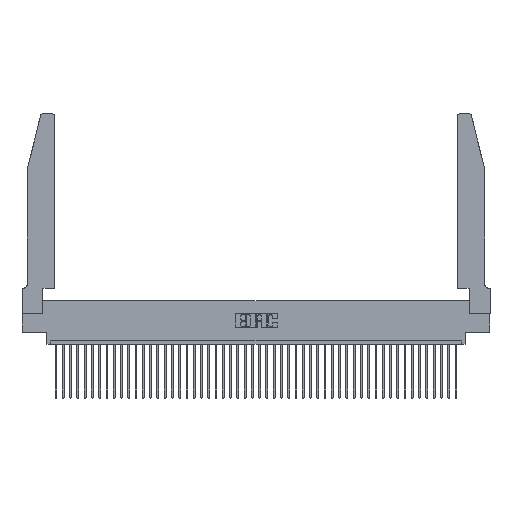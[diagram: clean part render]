
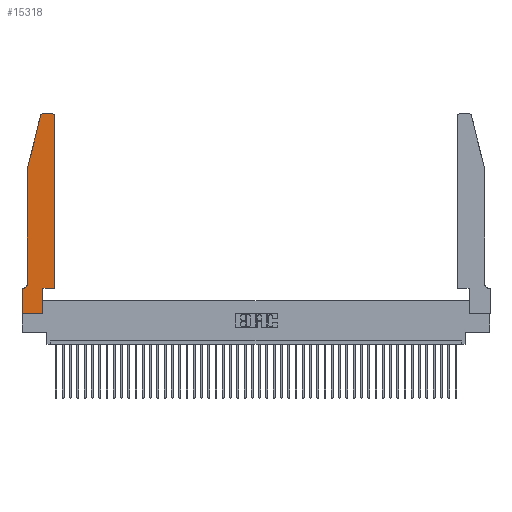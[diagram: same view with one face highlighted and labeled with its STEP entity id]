
A CAD part, top view. The second image highlights one B-rep face of the part: STEP entity #15318.
In plain terms, the highlighted planar face has unit normal (0, 0, 1).
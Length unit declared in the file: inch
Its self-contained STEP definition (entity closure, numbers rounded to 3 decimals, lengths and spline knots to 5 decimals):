
#3 = DIRECTION ( 'NONE',  ( 0., 1., 0. ) ) ;
#932 = DIRECTION ( 'NONE',  ( 0., -1., 0. ) ) ;
#965 = VECTOR ( 'NONE', #3, 39.37008 ) ;
#1330 = VERTEX_POINT ( 'NONE', #4524 ) ;
#2047 = ORIENTED_EDGE ( 'NONE', *, *, #10478, .T. ) ;
#2260 = LINE ( 'NONE', #42080, #41543 ) ;
#3039 = ORIENTED_EDGE ( 'NONE', *, *, #27211, .T. ) ;
#3111 = VERTEX_POINT ( 'NONE', #19077 ) ;
#3651 = LINE ( 'NONE', #14438, #29190 ) ;
#3782 = ORIENTED_EDGE ( 'NONE', *, *, #40038, .T. ) ;
#4115 = CARTESIAN_POINT ( 'NONE',  ( 0.0055, 0.35, 0.37 ) ) ;
#4524 = CARTESIAN_POINT ( 'NONE',  ( 0.25487, 2.72718, 0.37 ) ) ;
#4944 = EDGE_CURVE ( 'NONE', #32134, #42219, #15332, .T. ) ;
#6079 = CARTESIAN_POINT ( 'NONE',  ( 0.0755, 2., 0.37 ) ) ;
#6484 = EDGE_CURVE ( 'NONE', #40848, #12326, #9404, .T. ) ;
#7532 = CARTESIAN_POINT ( 'NONE',  ( 0.4505, 0.35, 0.37 ) ) ;
#8076 = DIRECTION ( 'NONE',  ( 0., 0., 1. ) ) ;
#8803 = ORIENTED_EDGE ( 'NONE', *, *, #30537, .T. ) ;
#9305 = ORIENTED_EDGE ( 'NONE', *, *, #6484, .T. ) ;
#9404 = LINE ( 'NONE', #20370, #38803 ) ;
#9510 = VERTEX_POINT ( 'NONE', #31432 ) ;
#9605 = CARTESIAN_POINT ( 'NONE',  ( 0.0055, 0.42, 0.37 ) ) ;
#9647 = VERTEX_POINT ( 'NONE', #38100 ) ;
#9669 = VECTOR ( 'NONE', #932, 39.37008 ) ;
#10478 = EDGE_CURVE ( 'NONE', #34378, #34641, #13978, .T. ) ;
#11453 = AXIS2_PLACEMENT_3D ( 'NONE', #23658, #41322, #34464 ) ;
#12167 = ORIENTED_EDGE ( 'NONE', *, *, #37083, .T. ) ;
#12326 = VERTEX_POINT ( 'NONE', #33422 ) ;
#13372 = CARTESIAN_POINT ( 'NONE',  ( 0., 0., 0.37 ) ) ;
#13695 = VECTOR ( 'NONE', #34147, 39.37008 ) ;
#13743 = ORIENTED_EDGE ( 'NONE', *, *, #31569, .T. ) ;
#13949 = DIRECTION ( 'NONE',  ( 0., 1., 0. ) ) ;
#13978 = CIRCLE ( 'NONE', #39617, 0.03 ) ;
#13996 = DIRECTION ( 'NONE',  ( 1., 0., 0. ) ) ;
#14005 = CARTESIAN_POINT ( 'NONE',  ( 0.2605, 2.75, 0.37 ) ) ;
#14438 = CARTESIAN_POINT ( 'NONE',  ( 0.0755, 2., 0.37 ) ) ;
#15318 = ADVANCED_FACE ( 'NONE', ( #31512 ), #33857, .T. ) ;
#15332 = LINE ( 'NONE', #20928, #13695 ) ;
#15644 = AXIS2_PLACEMENT_3D ( 'NONE', #9605, #44278, #34069 ) ;
#16637 = DIRECTION ( 'NONE',  ( 1., 0., 0. ) ) ;
#18770 = DIRECTION ( 'NONE',  ( 0., 0., 1. ) ) ;
#19077 = CARTESIAN_POINT ( 'NONE',  ( 0.284, 2.75, 0.37 ) ) ;
#20370 = CARTESIAN_POINT ( 'NONE',  ( 0.0755, 0.35, 0.37 ) ) ;
#20928 = CARTESIAN_POINT ( 'NONE',  ( 0., 0., 0.37 ) ) ;
#20960 = DIRECTION ( 'NONE',  ( -0.239, -0.971, 0. ) ) ;
#21564 = CARTESIAN_POINT ( 'NONE',  ( 0.284, 2.72, 0.37 ) ) ;
#21651 = CARTESIAN_POINT ( 'NONE',  ( 0.2865, 0.35, 0.37 ) ) ;
#22171 = LINE ( 'NONE', #35813, #9669 ) ;
#22509 = CARTESIAN_POINT ( 'NONE',  ( 0.4505, 2.72, 0.37 ) ) ;
#23502 = EDGE_CURVE ( 'NONE', #9510, #34378, #36922, .T. ) ;
#23594 = VECTOR ( 'NONE', #24025, 39.37008 ) ;
#23658 = CARTESIAN_POINT ( 'NONE',  ( 0., 0.35, 0.37 ) ) ;
#23957 = ORIENTED_EDGE ( 'NONE', *, *, #23502, .T. ) ;
#24025 = DIRECTION ( 'NONE',  ( -1., 0., 0. ) ) ;
#24248 = EDGE_CURVE ( 'NONE', #3111, #1330, #43454, .T. ) ;
#24462 = EDGE_CURVE ( 'NONE', #12326, #32134, #43469, .T. ) ;
#27211 = EDGE_CURVE ( 'NONE', #34641, #3111, #34525, .T. ) ;
#28226 = ORIENTED_EDGE ( 'NONE', *, *, #24248, .T. ) ;
#28287 = AXIS2_PLACEMENT_3D ( 'NONE', #21564, #18770, #16637 ) ;
#28865 = ORIENTED_EDGE ( 'NONE', *, *, #38122, .T. ) ;
#29190 = VECTOR ( 'NONE', #20960, 39.37008 ) ;
#30383 = CIRCLE ( 'NONE', #15644, 0.07 ) ;
#30537 = EDGE_CURVE ( 'NONE', #1330, #41046, #3651, .T. ) ;
#31432 = CARTESIAN_POINT ( 'NONE',  ( 0.4505, 0.35, 0.37 ) ) ;
#31512 = FACE_OUTER_BOUND ( 'NONE', #39662, .T. ) ;
#31569 = EDGE_CURVE ( 'NONE', #9647, #40848, #30383, .T. ) ;
#31606 = CARTESIAN_POINT ( 'NONE',  ( 0., 0., 0.37 ) ) ;
#32134 = VERTEX_POINT ( 'NONE', #13372 ) ;
#32686 = CARTESIAN_POINT ( 'NONE',  ( 0.4205, 2.72, 0.37 ) ) ;
#33422 = CARTESIAN_POINT ( 'NONE',  ( 0., 0.35, 0.37 ) ) ;
#33857 = PLANE ( 'NONE',  #11453 ) ;
#34069 = DIRECTION ( 'NONE',  ( -1., 0., 0. ) ) ;
#34147 = DIRECTION ( 'NONE',  ( 1., 0., 0. ) ) ;
#34378 = VERTEX_POINT ( 'NONE', #22509 ) ;
#34464 = DIRECTION ( 'NONE',  ( 1., 0., 0. ) ) ;
#34525 = LINE ( 'NONE', #14005, #23594 ) ;
#34641 = VERTEX_POINT ( 'NONE', #41523 ) ;
#34787 = VECTOR ( 'NONE', #39344, 39.37008 ) ;
#35813 = CARTESIAN_POINT ( 'NONE',  ( 0.0755, 2., 0.37 ) ) ;
#35886 = VERTEX_POINT ( 'NONE', #21651 ) ;
#36704 = ORIENTED_EDGE ( 'NONE', *, *, #24462, .T. ) ;
#36922 = LINE ( 'NONE', #7532, #965 ) ;
#37083 = EDGE_CURVE ( 'NONE', #41046, #9647, #22171, .T. ) ;
#37805 = CARTESIAN_POINT ( 'NONE',  ( 0.2865, 0., 0.37 ) ) ;
#38100 = CARTESIAN_POINT ( 'NONE',  ( 0.0755, 0.42, 0.37 ) ) ;
#38122 = EDGE_CURVE ( 'NONE', #35886, #9510, #42827, .T. ) ;
#38803 = VECTOR ( 'NONE', #41361, 39.37008 ) ;
#39344 = DIRECTION ( 'NONE',  ( 0., -1., 0. ) ) ;
#39617 = AXIS2_PLACEMENT_3D ( 'NONE', #32686, #8076, #39830 ) ;
#39662 = EDGE_LOOP ( 'NONE', ( #3039, #28226, #8803, #12167, #13743, #9305, #36704, #40674, #3782, #28865, #23957, #2047 ) ) ;
#39830 = DIRECTION ( 'NONE',  ( 1., 0., 0. ) ) ;
#40038 = EDGE_CURVE ( 'NONE', #42219, #35886, #2260, .T. ) ;
#40638 = VECTOR ( 'NONE', #13996, 39.37008 ) ;
#40674 = ORIENTED_EDGE ( 'NONE', *, *, #4944, .T. ) ;
#40848 = VERTEX_POINT ( 'NONE', #4115 ) ;
#41046 = VERTEX_POINT ( 'NONE', #6079 ) ;
#41322 = DIRECTION ( 'NONE',  ( 0., 0., 1. ) ) ;
#41361 = DIRECTION ( 'NONE',  ( -1., 0., 0. ) ) ;
#41523 = CARTESIAN_POINT ( 'NONE',  ( 0.4205, 2.75, 0.37 ) ) ;
#41543 = VECTOR ( 'NONE', #13949, 39.37008 ) ;
#42080 = CARTESIAN_POINT ( 'NONE',  ( 0.2865, 0.35, 0.37 ) ) ;
#42219 = VERTEX_POINT ( 'NONE', #37805 ) ;
#42827 = LINE ( 'NONE', #45023, #40638 ) ;
#43454 = CIRCLE ( 'NONE', #28287, 0.03 ) ;
#43469 = LINE ( 'NONE', #31606, #34787 ) ;
#44278 = DIRECTION ( 'NONE',  ( 0., 0., -1. ) ) ;
#45023 = CARTESIAN_POINT ( 'NONE',  ( 0.4505, 0.35, 0.37 ) ) ;
